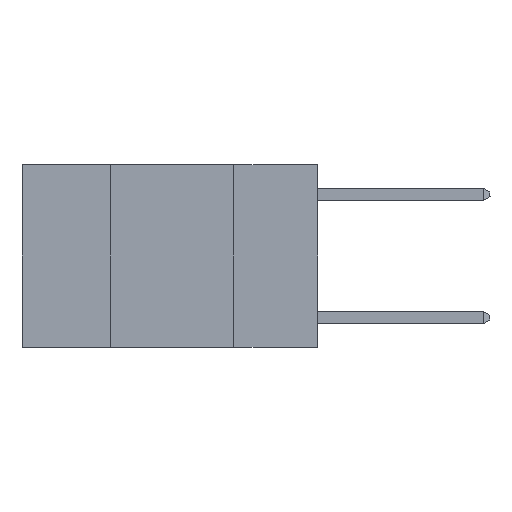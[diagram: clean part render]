
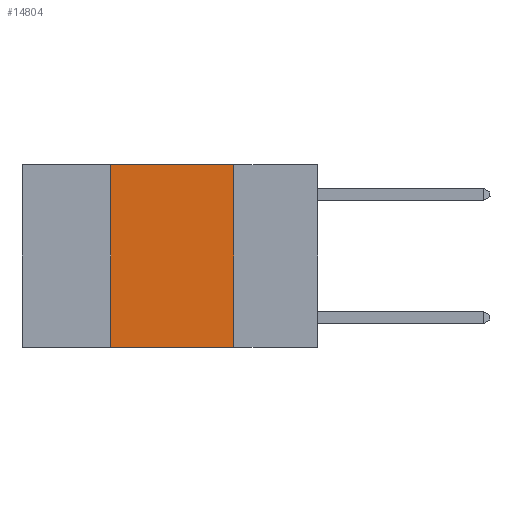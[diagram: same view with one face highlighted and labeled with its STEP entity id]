
A CAD part, left-side view. The second image highlights one B-rep face of the part: STEP entity #14804.
In plain terms, the highlighted planar face has unit normal (-1, 0, 0).
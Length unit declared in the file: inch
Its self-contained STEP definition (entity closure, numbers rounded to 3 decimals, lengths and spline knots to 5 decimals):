
#848 = DIRECTION ( 'NONE',  ( 0., 0., -1. ) ) ;
#973 = EDGE_CURVE ( 'NONE', #3634, #20307, #8744, .T. ) ;
#2266 = PLANE ( 'NONE',  #11126 ) ;
#2373 = DIRECTION ( 'NONE',  ( 0., 0., -1. ) ) ;
#2589 = ORIENTED_EDGE ( 'NONE', *, *, #973, .F. ) ;
#3634 = VERTEX_POINT ( 'NONE', #20025 ) ;
#3973 = VERTEX_POINT ( 'NONE', #14095 ) ;
#5018 = VECTOR ( 'NONE', #8111, 39.37008 ) ;
#5638 = EDGE_LOOP ( 'NONE', ( #11316, #17279, #2589, #6501 ) ) ;
#5830 = CARTESIAN_POINT ( 'NONE',  ( 0., 0.42, 0. ) ) ;
#6501 = ORIENTED_EDGE ( 'NONE', *, *, #12598, .T. ) ;
#6550 = CARTESIAN_POINT ( 'NONE',  ( 0., 0.6, 0. ) ) ;
#6882 = EDGE_CURVE ( 'NONE', #3973, #9186, #15176, .T. ) ;
#7330 = FACE_OUTER_BOUND ( 'NONE', #5638, .T. ) ;
#7669 = CARTESIAN_POINT ( 'NONE',  ( 0., 0.6, -0.37 ) ) ;
#8111 = DIRECTION ( 'NONE',  ( 0., -1., 0. ) ) ;
#8414 = VECTOR ( 'NONE', #15155, 39.37008 ) ;
#8744 = LINE ( 'NONE', #5830, #8414 ) ;
#9186 = VERTEX_POINT ( 'NONE', #11271 ) ;
#10239 = CARTESIAN_POINT ( 'NONE',  ( 0., 0.6, 0. ) ) ;
#11126 = AXIS2_PLACEMENT_3D ( 'NONE', #10239, #20037, #2373 ) ;
#11271 = CARTESIAN_POINT ( 'NONE',  ( 0., 0.17, -0.37 ) ) ;
#11316 = ORIENTED_EDGE ( 'NONE', *, *, #6882, .F. ) ;
#11686 = EDGE_CURVE ( 'NONE', #20307, #3973, #15987, .T. ) ;
#12598 = EDGE_CURVE ( 'NONE', #3634, #9186, #17515, .T. ) ;
#13357 = CARTESIAN_POINT ( 'NONE',  ( 0., 0.42, 0. ) ) ;
#14095 = CARTESIAN_POINT ( 'NONE',  ( 0., 0.17, 0. ) ) ;
#14804 = ADVANCED_FACE ( 'NONE', ( #7330 ), #2266, .F. ) ;
#15155 = DIRECTION ( 'NONE',  ( 0., 0., 1. ) ) ;
#15176 = LINE ( 'NONE', #20033, #16246 ) ;
#15987 = LINE ( 'NONE', #6550, #5018 ) ;
#16246 = VECTOR ( 'NONE', #848, 39.37008 ) ;
#17221 = DIRECTION ( 'NONE',  ( 0., -1., 0. ) ) ;
#17279 = ORIENTED_EDGE ( 'NONE', *, *, #11686, .F. ) ;
#17515 = LINE ( 'NONE', #7669, #19672 ) ;
#19672 = VECTOR ( 'NONE', #17221, 39.37008 ) ;
#20025 = CARTESIAN_POINT ( 'NONE',  ( 0., 0.42, -0.37 ) ) ;
#20033 = CARTESIAN_POINT ( 'NONE',  ( 0., 0.17, 0. ) ) ;
#20037 = DIRECTION ( 'NONE',  ( 1., 0., 0. ) ) ;
#20307 = VERTEX_POINT ( 'NONE', #13357 ) ;
